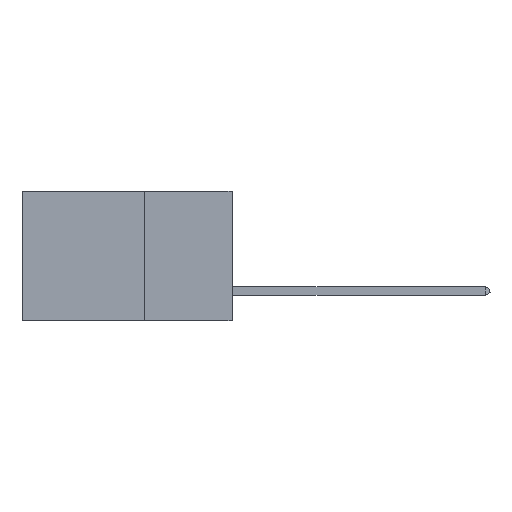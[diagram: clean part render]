
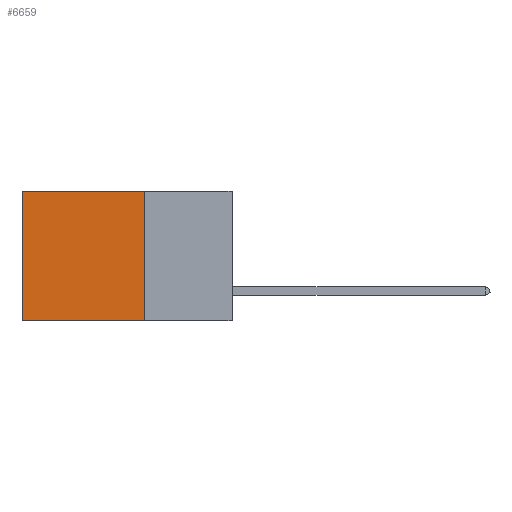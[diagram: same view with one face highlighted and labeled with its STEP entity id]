
A CAD part, left-side view. The second image highlights one B-rep face of the part: STEP entity #6659.
In plain terms, the highlighted planar face has unit normal (-1, 0, 0).
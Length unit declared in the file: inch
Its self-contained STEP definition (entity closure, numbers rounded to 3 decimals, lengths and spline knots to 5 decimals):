
#401 = CARTESIAN_POINT ( 'NONE',  ( 0.2875, 0.6, -0.37 ) ) ;
#463 = VERTEX_POINT ( 'NONE', #5355 ) ;
#595 = ORIENTED_EDGE ( 'NONE', *, *, #6111, .T. ) ;
#925 = VERTEX_POINT ( 'NONE', #401 ) ;
#1016 = PLANE ( 'NONE',  #14274 ) ;
#2384 = VERTEX_POINT ( 'NONE', #11402 ) ;
#2842 = VECTOR ( 'NONE', #11993, 39.37008 ) ;
#3657 = LINE ( 'NONE', #11607, #4712 ) ;
#3703 = ORIENTED_EDGE ( 'NONE', *, *, #5335, .F. ) ;
#4368 = EDGE_LOOP ( 'NONE', ( #6772, #9642, #3703, #595 ) ) ;
#4378 = LINE ( 'NONE', #9880, #2842 ) ;
#4712 = VECTOR ( 'NONE', #4956, 39.37008 ) ;
#4956 = DIRECTION ( 'NONE',  ( 0., 1., 0. ) ) ;
#5335 = EDGE_CURVE ( 'NONE', #8764, #463, #10129, .T. ) ;
#5355 = CARTESIAN_POINT ( 'NONE',  ( 0.2875, 0.25, -0.37 ) ) ;
#5396 = DIRECTION ( 'NONE',  ( 1., 0., 0. ) ) ;
#5649 = LINE ( 'NONE', #12720, #14112 ) ;
#6111 = EDGE_CURVE ( 'NONE', #8764, #2384, #4378, .T. ) ;
#6659 = ADVANCED_FACE ( 'NONE', ( #8487 ), #1016, .F. ) ;
#6772 = ORIENTED_EDGE ( 'NONE', *, *, #12083, .T. ) ;
#7209 = CARTESIAN_POINT ( 'NONE',  ( 0.2875, 0.25, 0. ) ) ;
#8059 = EDGE_CURVE ( 'NONE', #463, #925, #3657, .T. ) ;
#8487 = FACE_OUTER_BOUND ( 'NONE', #4368, .T. ) ;
#8656 = CARTESIAN_POINT ( 'NONE',  ( 0.2875, 0.25, 0. ) ) ;
#8764 = VERTEX_POINT ( 'NONE', #11701 ) ;
#9642 = ORIENTED_EDGE ( 'NONE', *, *, #8059, .F. ) ;
#9780 = VECTOR ( 'NONE', #10538, 39.37008 ) ;
#9880 = CARTESIAN_POINT ( 'NONE',  ( 0.2875, 0.25, 0. ) ) ;
#10129 = LINE ( 'NONE', #7209, #9780 ) ;
#10538 = DIRECTION ( 'NONE',  ( 0., 0., -1. ) ) ;
#11402 = CARTESIAN_POINT ( 'NONE',  ( 0.2875, 0.6, 0. ) ) ;
#11607 = CARTESIAN_POINT ( 'NONE',  ( 0.2875, 0.25, -0.37 ) ) ;
#11615 = DIRECTION ( 'NONE',  ( 0., 0., -1. ) ) ;
#11701 = CARTESIAN_POINT ( 'NONE',  ( 0.2875, 0.25, 0. ) ) ;
#11993 = DIRECTION ( 'NONE',  ( 0., 1., 0. ) ) ;
#12083 = EDGE_CURVE ( 'NONE', #2384, #925, #5649, .T. ) ;
#12720 = CARTESIAN_POINT ( 'NONE',  ( 0.2875, 0.6, 0. ) ) ;
#14112 = VECTOR ( 'NONE', #11615, 39.37008 ) ;
#14224 = DIRECTION ( 'NONE',  ( 0., 0., -1. ) ) ;
#14274 = AXIS2_PLACEMENT_3D ( 'NONE', #8656, #5396, #14224 ) ;
